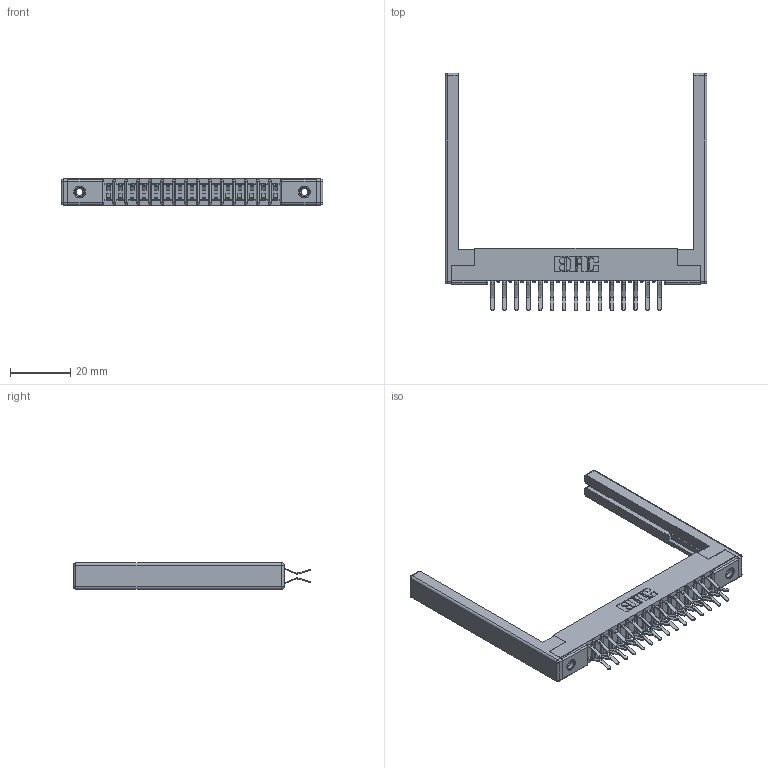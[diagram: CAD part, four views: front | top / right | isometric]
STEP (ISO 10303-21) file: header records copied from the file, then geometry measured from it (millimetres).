
FILE_DESCRIPTION (( 'STEP AP203' ), '1' );
FILE_NAME ('307-030-560-268.STEP', '2019-09-06T01:11:40', ( '' ), ( '' ), 'SwSTEP 2.0', 'SolidWorks 2016', '' );
FILE_SCHEMA (( 'CONFIG_CONTROL_DESIGN' ));
Length unit declared in the file: inch
Products named in the file (5): 307-290-001_560; 345-250-001_345-250-001-102; 307-030-560-268; 307-220-068; 307 Part_.156 Dia Mounting Holes
Assembly tree (35 placements, depth 2):
  307-030-560-268
    307 Part_.156 Dia Mounting Holes
    307-290-001_560  x30
    307-220-068  x2
    345-250-001_345-250-001-102  x2
Bounding box: 86.87 x 78.69 x 8.71 mm (x, y, z)
Volume: 10281.8 mm3; surface area: 14009.4 mm2
Topology: 35 solids, 35 shells, 1788 faces, 4973 edges, 3210 vertices
Faces by surface type: plane 1148, cylinder 584, sphere 40, cone 12, torus 4
Entity records: 19531 total; most frequent: CARTESIAN_POINT 3180, DIRECTION 3142, ORIENTED_EDGE 3140, EDGE_CURVE 1570, VECTOR 1190, LINE 1190, VERTEX_POINT 1014, AXIS2_PLACEMENT_3D 976
